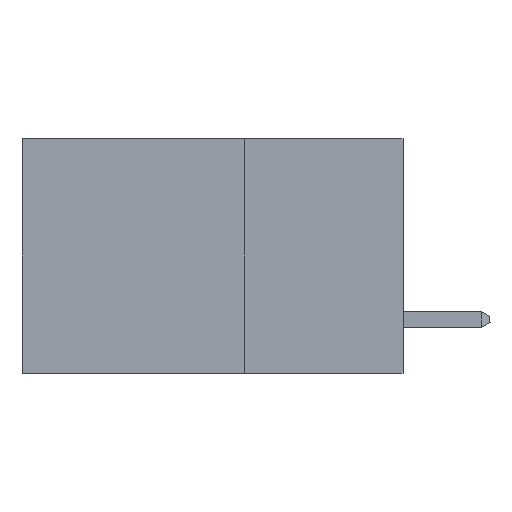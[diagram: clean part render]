
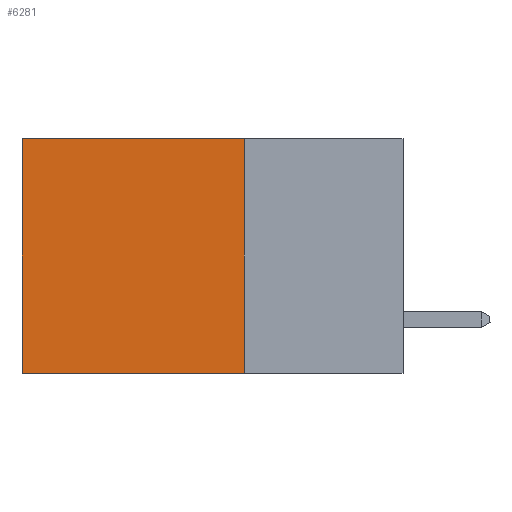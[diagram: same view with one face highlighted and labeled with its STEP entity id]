
A CAD part, left-side view. The second image highlights one B-rep face of the part: STEP entity #6281.
In plain terms, the highlighted planar face has unit normal (-1, 0, 0).
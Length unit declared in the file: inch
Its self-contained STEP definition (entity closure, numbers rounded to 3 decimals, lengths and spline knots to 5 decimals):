
#399 = PLANE ( 'NONE',  #15382 ) ;
#646 = VECTOR ( 'NONE', #31058, 39.37008 ) ;
#1476 = LINE ( 'NONE', #27821, #6081 ) ;
#5322 = ORIENTED_EDGE ( 'NONE', *, *, #13263, .T. ) ;
#5610 = DIRECTION ( 'NONE',  ( 0., 1., 0. ) ) ;
#6081 = VECTOR ( 'NONE', #18141, 39.37008 ) ;
#6281 = ADVANCED_FACE ( 'NONE', ( #8446 ), #399, .F. ) ;
#7325 = EDGE_CURVE ( 'NONE', #28934, #19748, #1476, .T. ) ;
#8446 = FACE_OUTER_BOUND ( 'NONE', #11214, .T. ) ;
#11214 = EDGE_LOOP ( 'NONE', ( #5322, #13017, #16672, #20982 ) ) ;
#12635 = LINE ( 'NONE', #17658, #21750 ) ;
#13017 = ORIENTED_EDGE ( 'NONE', *, *, #24850, .F. ) ;
#13045 = DIRECTION ( 'NONE',  ( 1., 0., 0. ) ) ;
#13263 = EDGE_CURVE ( 'NONE', #16001, #29816, #21669, .T. ) ;
#14340 = LINE ( 'NONE', #14785, #19269 ) ;
#14496 = DIRECTION ( 'NONE',  ( 0., 1., 0. ) ) ;
#14785 = CARTESIAN_POINT ( 'NONE',  ( 0.2875, 0.25, -0.37 ) ) ;
#15382 = AXIS2_PLACEMENT_3D ( 'NONE', #24349, #13045, #20356 ) ;
#16001 = VERTEX_POINT ( 'NONE', #21597 ) ;
#16127 = CARTESIAN_POINT ( 'NONE',  ( 0.2875, 0.6, 0. ) ) ;
#16672 = ORIENTED_EDGE ( 'NONE', *, *, #7325, .F. ) ;
#17658 = CARTESIAN_POINT ( 'NONE',  ( 0.2875, 0.25, 0. ) ) ;
#18141 = DIRECTION ( 'NONE',  ( 0., 0., -1. ) ) ;
#19269 = VECTOR ( 'NONE', #14496, 39.37008 ) ;
#19748 = VERTEX_POINT ( 'NONE', #31284 ) ;
#20356 = DIRECTION ( 'NONE',  ( 0., 0., -1. ) ) ;
#20982 = ORIENTED_EDGE ( 'NONE', *, *, #21602, .T. ) ;
#21597 = CARTESIAN_POINT ( 'NONE',  ( 0.2875, 0.6, 0. ) ) ;
#21602 = EDGE_CURVE ( 'NONE', #28934, #16001, #12635, .T. ) ;
#21669 = LINE ( 'NONE', #16127, #646 ) ;
#21750 = VECTOR ( 'NONE', #5610, 39.37008 ) ;
#24349 = CARTESIAN_POINT ( 'NONE',  ( 0.2875, 0.25, 0. ) ) ;
#24850 = EDGE_CURVE ( 'NONE', #19748, #29816, #14340, .T. ) ;
#27821 = CARTESIAN_POINT ( 'NONE',  ( 0.2875, 0.25, 0. ) ) ;
#28934 = VERTEX_POINT ( 'NONE', #30666 ) ;
#29220 = CARTESIAN_POINT ( 'NONE',  ( 0.2875, 0.6, -0.37 ) ) ;
#29816 = VERTEX_POINT ( 'NONE', #29220 ) ;
#30666 = CARTESIAN_POINT ( 'NONE',  ( 0.2875, 0.25, 0. ) ) ;
#31058 = DIRECTION ( 'NONE',  ( 0., 0., -1. ) ) ;
#31284 = CARTESIAN_POINT ( 'NONE',  ( 0.2875, 0.25, -0.37 ) ) ;
